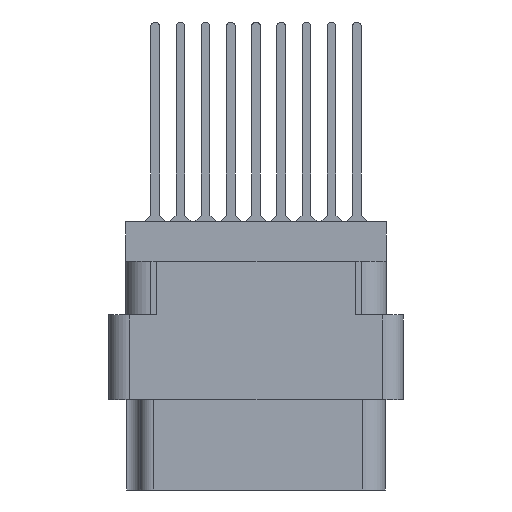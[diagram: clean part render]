
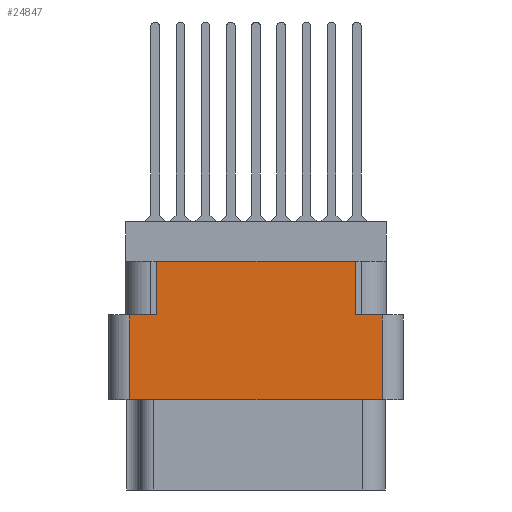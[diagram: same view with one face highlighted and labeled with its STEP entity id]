
A CAD part, left-side view. The second image highlights one B-rep face of the part: STEP entity #24847.
In plain terms, the highlighted planar face has unit normal (-1, 0, 0).
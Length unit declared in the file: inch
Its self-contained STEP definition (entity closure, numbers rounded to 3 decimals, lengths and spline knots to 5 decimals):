
#265 = VECTOR ( 'NONE', #43111, 39.37008 ) ;
#2594 = DIRECTION ( 'NONE',  ( 0., 1., 0. ) ) ;
#2953 = CARTESIAN_POINT ( 'NONE',  ( -1.296, 0., -0.529 ) ) ;
#3139 = ORIENTED_EDGE ( 'NONE', *, *, #44770, .F. ) ;
#3227 = ORIENTED_EDGE ( 'NONE', *, *, #47532, .T. ) ;
#3398 = EDGE_CURVE ( 'NONE', #32792, #13482, #50758, .T. ) ;
#3709 = EDGE_CURVE ( 'NONE', #14593, #9006, #16158, .T. ) ;
#4743 = CARTESIAN_POINT ( 'NONE',  ( -1.296, 0., -0.277 ) ) ;
#4876 = CARTESIAN_POINT ( 'NONE',  ( -1.296, -0.376, -0.798 ) ) ;
#5027 = ORIENTED_EDGE ( 'NONE', *, *, #42092, .F. ) ;
#5052 = VECTOR ( 'NONE', #50160, 39.37008 ) ;
#5682 = CARTESIAN_POINT ( 'NONE',  ( -1.296, -0.376, -0.277 ) ) ;
#6390 = CARTESIAN_POINT ( 'NONE',  ( -1.296, 0., -0.277 ) ) ;
#6961 = VECTOR ( 'NONE', #33070, 39.37008 ) ;
#7837 = CARTESIAN_POINT ( 'NONE',  ( -1.296, -0.296, -0.277 ) ) ;
#8212 = CARTESIAN_POINT ( 'NONE',  ( -1.296, -0.438, -0.798 ) ) ;
#8734 = ORIENTED_EDGE ( 'NONE', *, *, #3709, .F. ) ;
#9006 = VERTEX_POINT ( 'NONE', #34915 ) ;
#9114 = CARTESIAN_POINT ( 'NONE',  ( -1.296, 0.296, -0.277 ) ) ;
#9718 = CARTESIAN_POINT ( 'NONE',  ( -1.296, 0.376, -0.277 ) ) ;
#10396 = CARTESIAN_POINT ( 'NONE',  ( -1.296, 0.376, -0.798 ) ) ;
#11097 = VERTEX_POINT ( 'NONE', #5682 ) ;
#11687 = DIRECTION ( 'NONE',  ( 0., 0., 1. ) ) ;
#12282 = VECTOR ( 'NONE', #48749, 39.37008 ) ;
#13296 = VERTEX_POINT ( 'NONE', #7837 ) ;
#13482 = VERTEX_POINT ( 'NONE', #28203 ) ;
#13630 = VECTOR ( 'NONE', #2594, 39.37008 ) ;
#14436 = EDGE_CURVE ( 'NONE', #13296, #29617, #17560, .T. ) ;
#14516 = DIRECTION ( 'NONE',  ( 0., -1., 0. ) ) ;
#14593 = VERTEX_POINT ( 'NONE', #9718 ) ;
#15309 = ORIENTED_EDGE ( 'NONE', *, *, #14436, .T. ) ;
#15728 = DIRECTION ( 'NONE',  ( 0., 0., 1. ) ) ;
#16158 = LINE ( 'NONE', #6390, #34618 ) ;
#17438 = LINE ( 'NONE', #4743, #39105 ) ;
#17560 = LINE ( 'NONE', #31150, #265 ) ;
#19520 = DIRECTION ( 'NONE',  ( -1., 0., 0. ) ) ;
#19986 = LINE ( 'NONE', #28797, #6961 ) ;
#21921 = VECTOR ( 'NONE', #15728, 39.37008 ) ;
#23471 = ORIENTED_EDGE ( 'NONE', *, *, #49496, .F. ) ;
#24006 = CARTESIAN_POINT ( 'NONE',  ( -1.296, -0.296, -0.117 ) ) ;
#24847 = ADVANCED_FACE ( 'NONE', ( #36696 ), #50928, .T. ) ;
#28203 = CARTESIAN_POINT ( 'NONE',  ( -1.296, 0.376, -0.529 ) ) ;
#28376 = DIRECTION ( 'NONE',  ( 0., -1., 0. ) ) ;
#28797 = CARTESIAN_POINT ( 'NONE',  ( -1.296, 0.438, -0.117 ) ) ;
#29617 = VERTEX_POINT ( 'NONE', #24006 ) ;
#29632 = CARTESIAN_POINT ( 'NONE',  ( -1.296, 0.296, -0.117 ) ) ;
#31150 = CARTESIAN_POINT ( 'NONE',  ( -1.296, -0.296, -0.277 ) ) ;
#32792 = VERTEX_POINT ( 'NONE', #33902 ) ;
#33070 = DIRECTION ( 'NONE',  ( 0., -1., 0. ) ) ;
#33292 = EDGE_LOOP ( 'NONE', ( #8734, #41894, #47186, #3227, #23471, #15309, #5027, #3139 ) ) ;
#33902 = CARTESIAN_POINT ( 'NONE',  ( -1.296, -0.376, -0.529 ) ) ;
#34618 = VECTOR ( 'NONE', #14516, 39.37008 ) ;
#34834 = LINE ( 'NONE', #9114, #21921 ) ;
#34915 = CARTESIAN_POINT ( 'NONE',  ( -1.296, 0.296, -0.277 ) ) ;
#36696 = FACE_OUTER_BOUND ( 'NONE', #33292, .T. ) ;
#36928 = AXIS2_PLACEMENT_3D ( 'NONE', #8212, #19520, #11687 ) ;
#38006 = VERTEX_POINT ( 'NONE', #29632 ) ;
#39105 = VECTOR ( 'NONE', #28376, 39.37008 ) ;
#41894 = ORIENTED_EDGE ( 'NONE', *, *, #49810, .T. ) ;
#42092 = EDGE_CURVE ( 'NONE', #38006, #29617, #19986, .T. ) ;
#43111 = DIRECTION ( 'NONE',  ( 0., 0., 1. ) ) ;
#43798 = LINE ( 'NONE', #4876, #12282 ) ;
#44770 = EDGE_CURVE ( 'NONE', #9006, #38006, #34834, .T. ) ;
#45845 = LINE ( 'NONE', #10396, #5052 ) ;
#47186 = ORIENTED_EDGE ( 'NONE', *, *, #3398, .F. ) ;
#47532 = EDGE_CURVE ( 'NONE', #32792, #11097, #43798, .T. ) ;
#48749 = DIRECTION ( 'NONE',  ( 0., 0., 1. ) ) ;
#49496 = EDGE_CURVE ( 'NONE', #13296, #11097, #17438, .T. ) ;
#49810 = EDGE_CURVE ( 'NONE', #14593, #13482, #45845, .T. ) ;
#50160 = DIRECTION ( 'NONE',  ( 0., 0., -1. ) ) ;
#50758 = LINE ( 'NONE', #2953, #13630 ) ;
#50928 = PLANE ( 'NONE',  #36928 ) ;
